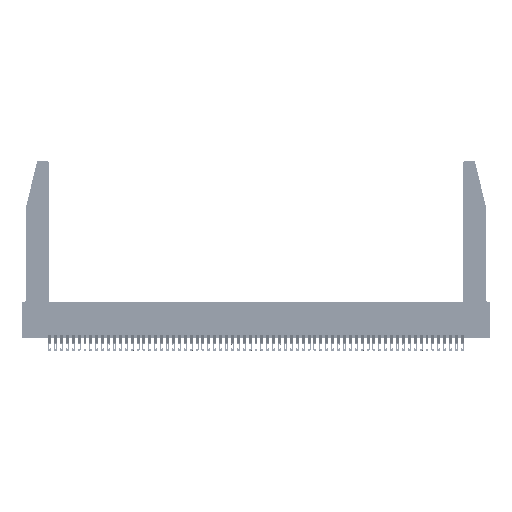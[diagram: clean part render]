
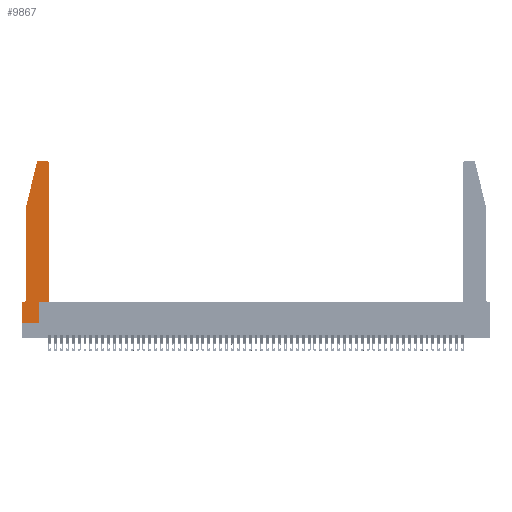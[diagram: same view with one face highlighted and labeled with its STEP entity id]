
A CAD part, top view. The second image highlights one B-rep face of the part: STEP entity #9867.
In plain terms, the highlighted planar face has unit normal (0, 0, 1).
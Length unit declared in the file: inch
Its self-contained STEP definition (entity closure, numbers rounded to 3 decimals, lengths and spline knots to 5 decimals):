
#25 = VECTOR ( 'NONE', #48573, 39.37008 ) ;
#378 = CARTESIAN_POINT ( 'NONE',  ( 0.4505, 0.35, 0.37 ) ) ;
#394 = LINE ( 'NONE', #38057, #29972 ) ;
#595 = DIRECTION ( 'NONE',  ( 0., 1., 0. ) ) ;
#894 = VERTEX_POINT ( 'NONE', #8610 ) ;
#1272 = CIRCLE ( 'NONE', #42636, 0.03 ) ;
#3001 = LINE ( 'NONE', #26916, #9170 ) ;
#3074 = CARTESIAN_POINT ( 'NONE',  ( 0.4505, 2.72, 0.37 ) ) ;
#3148 = DIRECTION ( 'NONE',  ( 1., 0., 0. ) ) ;
#3615 = ORIENTED_EDGE ( 'NONE', *, *, #55001, .T. ) ;
#4385 = LINE ( 'NONE', #4850, #6436 ) ;
#4850 = CARTESIAN_POINT ( 'NONE',  ( 0.2605, 2.75, 0.37 ) ) ;
#5806 = EDGE_CURVE ( 'NONE', #52649, #6131, #35743, .T. ) ;
#5832 = VECTOR ( 'NONE', #36334, 39.37008 ) ;
#6131 = VERTEX_POINT ( 'NONE', #33675 ) ;
#6436 = VECTOR ( 'NONE', #9864, 39.37008 ) ;
#7416 = VERTEX_POINT ( 'NONE', #25046 ) ;
#7845 = EDGE_CURVE ( 'NONE', #28607, #40496, #1272, .T. ) ;
#8432 = ORIENTED_EDGE ( 'NONE', *, *, #7845, .T. ) ;
#8485 = EDGE_CURVE ( 'NONE', #37118, #40098, #10088, .T. ) ;
#8610 = CARTESIAN_POINT ( 'NONE',  ( 0.2865, 0.35, 0.37 ) ) ;
#8897 = CARTESIAN_POINT ( 'NONE',  ( 0.0055, 0.35, 0.37 ) ) ;
#9128 = AXIS2_PLACEMENT_3D ( 'NONE', #20484, #12027, #3148 ) ;
#9170 = VECTOR ( 'NONE', #595, 39.37008 ) ;
#9390 = CARTESIAN_POINT ( 'NONE',  ( 0.2865, 0., 0.37 ) ) ;
#9646 = LINE ( 'NONE', #53185, #25 ) ;
#9799 = CARTESIAN_POINT ( 'NONE',  ( 0.4205, 2.72, 0.37 ) ) ;
#9864 = DIRECTION ( 'NONE',  ( -1., 0., 0. ) ) ;
#9867 = ADVANCED_FACE ( 'NONE', ( #56041 ), #37111, .T. ) ;
#9987 = DIRECTION ( 'NONE',  ( 1., 0., 0. ) ) ;
#10088 = CIRCLE ( 'NONE', #38243, 0.07 ) ;
#10197 = DIRECTION ( 'NONE',  ( 1., 0., 0. ) ) ;
#10374 = EDGE_CURVE ( 'NONE', #40496, #7416, #4385, .T. ) ;
#11932 = DIRECTION ( 'NONE',  ( 1., 0., 0. ) ) ;
#12027 = DIRECTION ( 'NONE',  ( 0., 0., 1. ) ) ;
#12141 = CARTESIAN_POINT ( 'NONE',  ( 0., 0., 0.37 ) ) ;
#12254 = EDGE_CURVE ( 'NONE', #40098, #26012, #9646, .T. ) ;
#14210 = EDGE_CURVE ( 'NONE', #26012, #49326, #33482, .T. ) ;
#15237 = VERTEX_POINT ( 'NONE', #25978 ) ;
#15414 = DIRECTION ( 'NONE',  ( 0., 0., 1. ) ) ;
#16233 = CARTESIAN_POINT ( 'NONE',  ( 0., 0.35, 0.37 ) ) ;
#19053 = CARTESIAN_POINT ( 'NONE',  ( 0., 0.35, 0.37 ) ) ;
#19732 = VECTOR ( 'NONE', #41473, 39.37008 ) ;
#20484 = CARTESIAN_POINT ( 'NONE',  ( 0.284, 2.72, 0.37 ) ) ;
#20794 = AXIS2_PLACEMENT_3D ( 'NONE', #19053, #15414, #10197 ) ;
#24390 = LINE ( 'NONE', #55602, #48415 ) ;
#25046 = CARTESIAN_POINT ( 'NONE',  ( 0.284, 2.75, 0.37 ) ) ;
#25814 = ORIENTED_EDGE ( 'NONE', *, *, #47607, .T. ) ;
#25978 = CARTESIAN_POINT ( 'NONE',  ( 0.4505, 0.35, 0.37 ) ) ;
#26012 = VERTEX_POINT ( 'NONE', #16233 ) ;
#26916 = CARTESIAN_POINT ( 'NONE',  ( 0.4505, 0.35, 0.37 ) ) ;
#26998 = CIRCLE ( 'NONE', #9128, 0.03 ) ;
#27076 = ORIENTED_EDGE ( 'NONE', *, *, #14210, .T. ) ;
#27690 = DIRECTION ( 'NONE',  ( -0.239, -0.971, 0. ) ) ;
#27937 = EDGE_CURVE ( 'NONE', #7416, #52649, #26998, .T. ) ;
#28549 = CARTESIAN_POINT ( 'NONE',  ( 0., 0., 0.37 ) ) ;
#28607 = VERTEX_POINT ( 'NONE', #3074 ) ;
#28647 = DIRECTION ( 'NONE',  ( 0., -1., 0. ) ) ;
#29972 = VECTOR ( 'NONE', #11932, 39.37008 ) ;
#30431 = CARTESIAN_POINT ( 'NONE',  ( 0.4205, 2.75, 0.37 ) ) ;
#31635 = CARTESIAN_POINT ( 'NONE',  ( 0.0755, 0.42, 0.37 ) ) ;
#31801 = ORIENTED_EDGE ( 'NONE', *, *, #40291, .T. ) ;
#31955 = CARTESIAN_POINT ( 'NONE',  ( 0.0755, 2., 0.37 ) ) ;
#33482 = LINE ( 'NONE', #28549, #19732 ) ;
#33675 = CARTESIAN_POINT ( 'NONE',  ( 0.0755, 2., 0.37 ) ) ;
#34013 = EDGE_LOOP ( 'NONE', ( #46268, #35234, #43596, #39207, #34506, #38552, #27076, #3615, #31801, #55245, #25814, #8432 ) ) ;
#34506 = ORIENTED_EDGE ( 'NONE', *, *, #8485, .T. ) ;
#35234 = ORIENTED_EDGE ( 'NONE', *, *, #27937, .T. ) ;
#35743 = LINE ( 'NONE', #31955, #46761 ) ;
#36334 = DIRECTION ( 'NONE',  ( 1., 0., 0. ) ) ;
#36658 = VECTOR ( 'NONE', #28647, 39.37008 ) ;
#37111 = PLANE ( 'NONE',  #20794 ) ;
#37118 = VERTEX_POINT ( 'NONE', #31635 ) ;
#37995 = EDGE_CURVE ( 'NONE', #6131, #37118, #52469, .T. ) ;
#38057 = CARTESIAN_POINT ( 'NONE',  ( 0., 0., 0.37 ) ) ;
#38243 = AXIS2_PLACEMENT_3D ( 'NONE', #44565, #48953, #53371 ) ;
#38552 = ORIENTED_EDGE ( 'NONE', *, *, #12254, .T. ) ;
#39207 = ORIENTED_EDGE ( 'NONE', *, *, #37995, .T. ) ;
#40098 = VERTEX_POINT ( 'NONE', #8897 ) ;
#40291 = EDGE_CURVE ( 'NONE', #49545, #894, #24390, .T. ) ;
#40496 = VERTEX_POINT ( 'NONE', #30431 ) ;
#40965 = DIRECTION ( 'NONE',  ( 0., 0., 1. ) ) ;
#41473 = DIRECTION ( 'NONE',  ( 0., -1., 0. ) ) ;
#42636 = AXIS2_PLACEMENT_3D ( 'NONE', #9799, #40965, #9987 ) ;
#43596 = ORIENTED_EDGE ( 'NONE', *, *, #5806, .T. ) ;
#44565 = CARTESIAN_POINT ( 'NONE',  ( 0.0055, 0.42, 0.37 ) ) ;
#46268 = ORIENTED_EDGE ( 'NONE', *, *, #10374, .T. ) ;
#46540 = CARTESIAN_POINT ( 'NONE',  ( 0.0755, 2., 0.37 ) ) ;
#46761 = VECTOR ( 'NONE', #27690, 39.37008 ) ;
#47607 = EDGE_CURVE ( 'NONE', #15237, #28607, #3001, .T. ) ;
#48415 = VECTOR ( 'NONE', #51374, 39.37008 ) ;
#48573 = DIRECTION ( 'NONE',  ( -1., 0., 0. ) ) ;
#48953 = DIRECTION ( 'NONE',  ( 0., 0., -1. ) ) ;
#49326 = VERTEX_POINT ( 'NONE', #12141 ) ;
#49545 = VERTEX_POINT ( 'NONE', #9390 ) ;
#49864 = LINE ( 'NONE', #378, #5832 ) ;
#50795 = CARTESIAN_POINT ( 'NONE',  ( 0.25487, 2.72718, 0.37 ) ) ;
#51374 = DIRECTION ( 'NONE',  ( 0., 1., 0. ) ) ;
#52469 = LINE ( 'NONE', #46540, #36658 ) ;
#52649 = VERTEX_POINT ( 'NONE', #50795 ) ;
#53185 = CARTESIAN_POINT ( 'NONE',  ( 0.0755, 0.35, 0.37 ) ) ;
#53371 = DIRECTION ( 'NONE',  ( -1., 0., 0. ) ) ;
#55001 = EDGE_CURVE ( 'NONE', #49326, #49545, #394, .T. ) ;
#55179 = EDGE_CURVE ( 'NONE', #894, #15237, #49864, .T. ) ;
#55245 = ORIENTED_EDGE ( 'NONE', *, *, #55179, .T. ) ;
#55602 = CARTESIAN_POINT ( 'NONE',  ( 0.2865, 0.35, 0.37 ) ) ;
#56041 = FACE_OUTER_BOUND ( 'NONE', #34013, .T. ) ;
